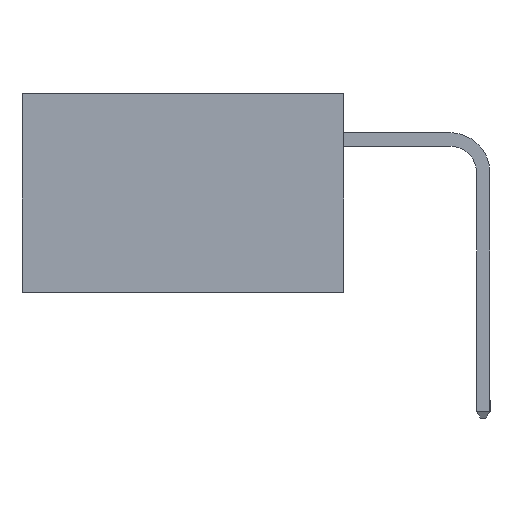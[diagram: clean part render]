
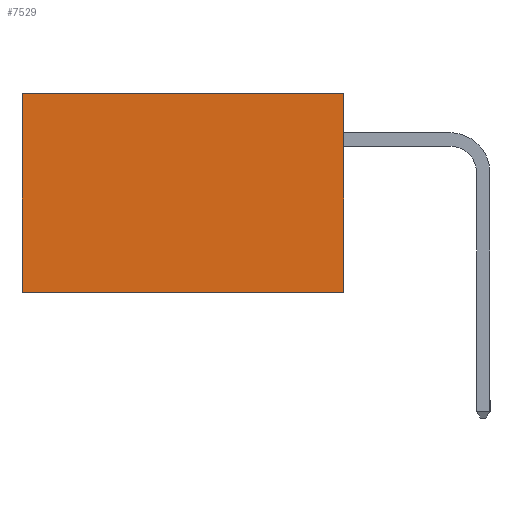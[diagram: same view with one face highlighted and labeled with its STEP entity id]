
A CAD part, left-side view. The second image highlights one B-rep face of the part: STEP entity #7529.
In plain terms, the highlighted planar face has unit normal (-1, 0, 0).
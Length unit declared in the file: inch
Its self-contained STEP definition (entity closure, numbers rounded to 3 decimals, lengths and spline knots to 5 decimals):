
#585 = CARTESIAN_POINT ( 'NONE',  ( 0.2615, 0.6, 0. ) ) ;
#1800 = DIRECTION ( 'NONE',  ( 0., 1., 0. ) ) ;
#2037 = CARTESIAN_POINT ( 'NONE',  ( 0.2615, 0., -0.37 ) ) ;
#2807 = ORIENTED_EDGE ( 'NONE', *, *, #13981, .F. ) ;
#3030 = EDGE_LOOP ( 'NONE', ( #9755, #9316, #2807, #10428 ) ) ;
#3496 = LINE ( 'NONE', #2037, #15176 ) ;
#3575 = DIRECTION ( 'NONE',  ( 0., 0., -1. ) ) ;
#5031 = CARTESIAN_POINT ( 'NONE',  ( 0.2615, 0., 0. ) ) ;
#5684 = CARTESIAN_POINT ( 'NONE',  ( 0.2615, 0.6, -0.37 ) ) ;
#6698 = DIRECTION ( 'NONE',  ( 0., 1., 0. ) ) ;
#6900 = PLANE ( 'NONE',  #9334 ) ;
#7454 = CARTESIAN_POINT ( 'NONE',  ( 0.2615, 0., -0.37 ) ) ;
#7529 = ADVANCED_FACE ( 'NONE', ( #8936 ), #6900, .F. ) ;
#8167 = VECTOR ( 'NONE', #1800, 39.37008 ) ;
#8936 = FACE_OUTER_BOUND ( 'NONE', #3030, .T. ) ;
#9316 = ORIENTED_EDGE ( 'NONE', *, *, #16636, .F. ) ;
#9334 = AXIS2_PLACEMENT_3D ( 'NONE', #17492, #19031, #9954 ) ;
#9486 = EDGE_CURVE ( 'NONE', #14593, #12137, #16535, .T. ) ;
#9670 = VERTEX_POINT ( 'NONE', #5684 ) ;
#9755 = ORIENTED_EDGE ( 'NONE', *, *, #18821, .T. ) ;
#9954 = DIRECTION ( 'NONE',  ( 0., 0., -1. ) ) ;
#10428 = ORIENTED_EDGE ( 'NONE', *, *, #9486, .T. ) ;
#11435 = VECTOR ( 'NONE', #13350, 39.37008 ) ;
#11810 = CARTESIAN_POINT ( 'NONE',  ( 0.2615, 0.6, -0.37 ) ) ;
#12137 = VERTEX_POINT ( 'NONE', #585 ) ;
#12223 = LINE ( 'NONE', #17010, #8167 ) ;
#12449 = VERTEX_POINT ( 'NONE', #7454 ) ;
#12534 = VECTOR ( 'NONE', #6698, 39.37008 ) ;
#13350 = DIRECTION ( 'NONE',  ( 0., 0., -1. ) ) ;
#13981 = EDGE_CURVE ( 'NONE', #14593, #12449, #3496, .T. ) ;
#14593 = VERTEX_POINT ( 'NONE', #5031 ) ;
#15176 = VECTOR ( 'NONE', #3575, 39.37008 ) ;
#15471 = LINE ( 'NONE', #11810, #11435 ) ;
#16535 = LINE ( 'NONE', #17287, #12534 ) ;
#16636 = EDGE_CURVE ( 'NONE', #12449, #9670, #12223, .T. ) ;
#17010 = CARTESIAN_POINT ( 'NONE',  ( 0.2615, 0., -0.37 ) ) ;
#17287 = CARTESIAN_POINT ( 'NONE',  ( 0.2615, 0., 0. ) ) ;
#17492 = CARTESIAN_POINT ( 'NONE',  ( 0.2615, 0., -0.37 ) ) ;
#18821 = EDGE_CURVE ( 'NONE', #12137, #9670, #15471, .T. ) ;
#19031 = DIRECTION ( 'NONE',  ( 1., 0., 0. ) ) ;
